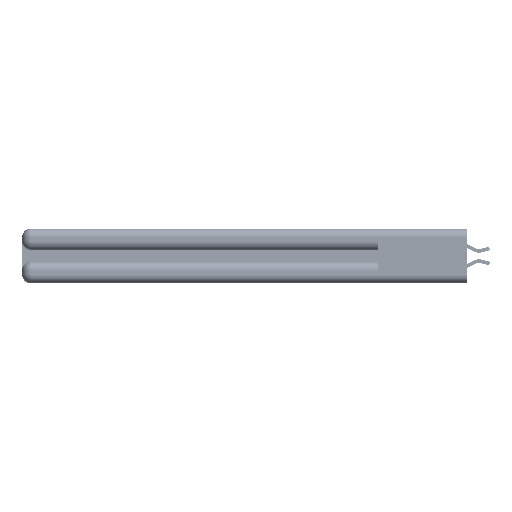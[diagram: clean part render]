
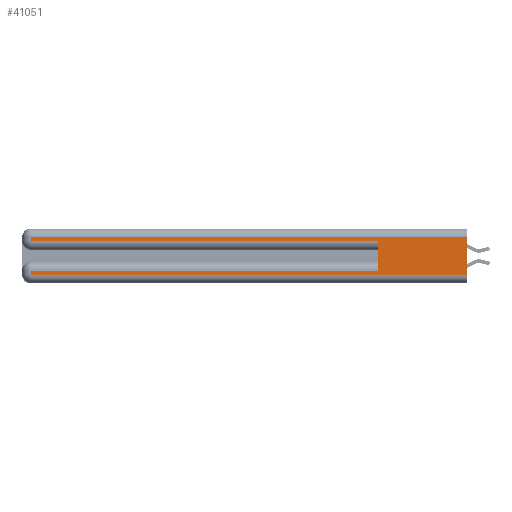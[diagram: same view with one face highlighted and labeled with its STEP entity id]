
A CAD part, left-side view. The second image highlights one B-rep face of the part: STEP entity #41051.
In plain terms, the highlighted planar face has unit normal (-1, 0, 0).
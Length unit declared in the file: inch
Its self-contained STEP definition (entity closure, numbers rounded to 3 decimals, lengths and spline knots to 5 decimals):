
#204 = VERTEX_POINT ( 'NONE', #13637 ) ;
#417 = LINE ( 'NONE', #23403, #24130 ) ;
#697 = ORIENTED_EDGE ( 'NONE', *, *, #14692, .T. ) ;
#1229 = CARTESIAN_POINT ( 'NONE',  ( 0., 0., 0.06 ) ) ;
#1675 = CARTESIAN_POINT ( 'NONE',  ( 0., 0., 0.06 ) ) ;
#2106 = ORIENTED_EDGE ( 'NONE', *, *, #8554, .F. ) ;
#3702 = AXIS2_PLACEMENT_3D ( 'NONE', #15139, #19657, #50451 ) ;
#5652 = ORIENTED_EDGE ( 'NONE', *, *, #17440, .T. ) ;
#6112 = VERTEX_POINT ( 'NONE', #20677 ) ;
#6986 = ORIENTED_EDGE ( 'NONE', *, *, #40293, .F. ) ;
#8483 = VECTOR ( 'NONE', #53650, 39.37008 ) ;
#8554 = EDGE_CURVE ( 'NONE', #9576, #17591, #10566, .T. ) ;
#8642 = CARTESIAN_POINT ( 'NONE',  ( 0., 0.6, 0.085 ) ) ;
#9006 = LINE ( 'NONE', #24630, #42933 ) ;
#9067 = CARTESIAN_POINT ( 'NONE',  ( 0., 2.94, 0.085 ) ) ;
#9576 = VERTEX_POINT ( 'NONE', #23532 ) ;
#9963 = DIRECTION ( 'NONE',  ( 0., 1., 0. ) ) ;
#10566 = LINE ( 'NONE', #14111, #23810 ) ;
#11925 = ORIENTED_EDGE ( 'NONE', *, *, #34593, .T. ) ;
#12881 = LINE ( 'NONE', #32469, #46739 ) ;
#13120 = VECTOR ( 'NONE', #28317, 39.37008 ) ;
#13198 = CARTESIAN_POINT ( 'NONE',  ( 0., 0., 0.285 ) ) ;
#13507 = EDGE_CURVE ( 'NONE', #55586, #17591, #36733, .T. ) ;
#13637 = CARTESIAN_POINT ( 'NONE',  ( 0., 2.94, 0.285 ) ) ;
#14111 = CARTESIAN_POINT ( 'NONE',  ( 0., 0., 0.37 ) ) ;
#14692 = EDGE_CURVE ( 'NONE', #49339, #23877, #417, .T. ) ;
#15139 = CARTESIAN_POINT ( 'NONE',  ( 0., 0., 0.37 ) ) ;
#15151 = CARTESIAN_POINT ( 'NONE',  ( 0., 2.94, 0.37 ) ) ;
#15231 = LINE ( 'NONE', #13198, #37427 ) ;
#16784 = ORIENTED_EDGE ( 'NONE', *, *, #35871, .T. ) ;
#17440 = EDGE_CURVE ( 'NONE', #24088, #204, #20335, .T. ) ;
#17591 = VERTEX_POINT ( 'NONE', #1229 ) ;
#18430 = CARTESIAN_POINT ( 'NONE',  ( 0., 2.94, 0.37 ) ) ;
#19657 = DIRECTION ( 'NONE',  ( 1., 0., 0. ) ) ;
#20335 = LINE ( 'NONE', #18430, #8483 ) ;
#20677 = CARTESIAN_POINT ( 'NONE',  ( 0., 0.6, 0.285 ) ) ;
#23403 = CARTESIAN_POINT ( 'NONE',  ( 0., 0., 0.085 ) ) ;
#23532 = CARTESIAN_POINT ( 'NONE',  ( 0., 0., 0.31 ) ) ;
#23810 = VECTOR ( 'NONE', #45001, 39.37008 ) ;
#23877 = VERTEX_POINT ( 'NONE', #9067 ) ;
#24088 = VERTEX_POINT ( 'NONE', #24435 ) ;
#24130 = VECTOR ( 'NONE', #9963, 39.37008 ) ;
#24435 = CARTESIAN_POINT ( 'NONE',  ( 0., 2.94, 0.31 ) ) ;
#24630 = CARTESIAN_POINT ( 'NONE',  ( 0., 0., 0.31 ) ) ;
#28317 = DIRECTION ( 'NONE',  ( 0., -1., 0. ) ) ;
#29058 = DIRECTION ( 'NONE',  ( 0., 1., 0. ) ) ;
#31788 = EDGE_LOOP ( 'NONE', ( #2106, #11925, #5652, #42977, #6986, #697, #16784, #32073 ) ) ;
#32073 = ORIENTED_EDGE ( 'NONE', *, *, #13507, .T. ) ;
#32469 = CARTESIAN_POINT ( 'NONE',  ( 0., 0.6, 0.145 ) ) ;
#34593 = EDGE_CURVE ( 'NONE', #9576, #24088, #9006, .T. ) ;
#35871 = EDGE_CURVE ( 'NONE', #23877, #55586, #38799, .T. ) ;
#36733 = LINE ( 'NONE', #1675, #13120 ) ;
#37266 = DIRECTION ( 'NONE',  ( 0., 0., -1. ) ) ;
#37427 = VECTOR ( 'NONE', #39728, 39.37008 ) ;
#38799 = LINE ( 'NONE', #15151, #49056 ) ;
#39728 = DIRECTION ( 'NONE',  ( 0., -1., 0. ) ) ;
#40293 = EDGE_CURVE ( 'NONE', #49339, #6112, #12881, .T. ) ;
#41051 = ADVANCED_FACE ( 'NONE', ( #48738 ), #46005, .F. ) ;
#42933 = VECTOR ( 'NONE', #29058, 39.37008 ) ;
#42977 = ORIENTED_EDGE ( 'NONE', *, *, #45138, .T. ) ;
#45001 = DIRECTION ( 'NONE',  ( 0., 0., -1. ) ) ;
#45138 = EDGE_CURVE ( 'NONE', #204, #6112, #15231, .T. ) ;
#45331 = CARTESIAN_POINT ( 'NONE',  ( 0., 2.94, 0.06 ) ) ;
#46005 = PLANE ( 'NONE',  #3702 ) ;
#46739 = VECTOR ( 'NONE', #54157, 39.37008 ) ;
#48738 = FACE_OUTER_BOUND ( 'NONE', #31788, .T. ) ;
#49056 = VECTOR ( 'NONE', #37266, 39.37008 ) ;
#49339 = VERTEX_POINT ( 'NONE', #8642 ) ;
#50451 = DIRECTION ( 'NONE',  ( 0., 0., -1. ) ) ;
#53650 = DIRECTION ( 'NONE',  ( 0., 0., -1. ) ) ;
#54157 = DIRECTION ( 'NONE',  ( 0., 0., 1. ) ) ;
#55586 = VERTEX_POINT ( 'NONE', #45331 ) ;
